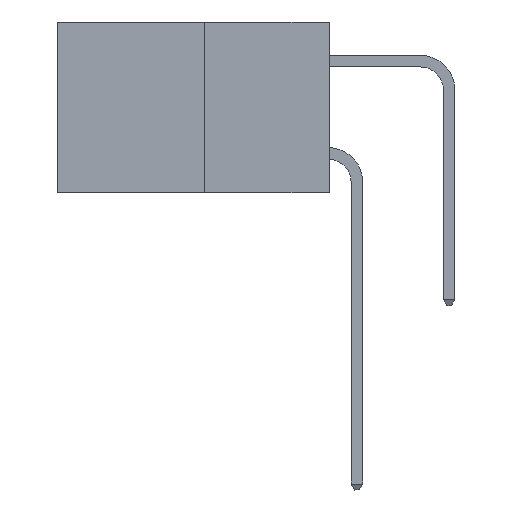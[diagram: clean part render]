
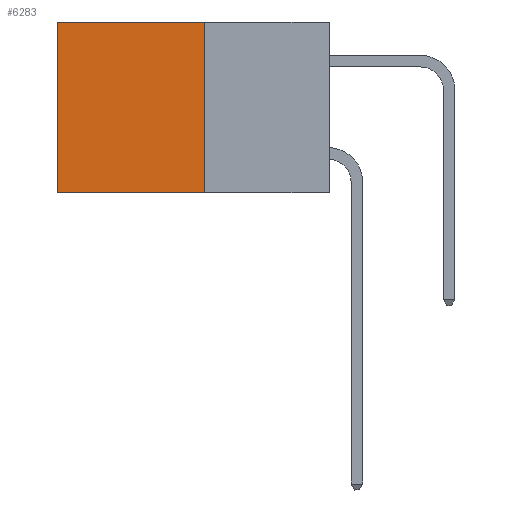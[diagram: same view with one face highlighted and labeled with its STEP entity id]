
A CAD part, left-side view. The second image highlights one B-rep face of the part: STEP entity #6283.
In plain terms, the highlighted planar face has unit normal (-1, 0, 0).
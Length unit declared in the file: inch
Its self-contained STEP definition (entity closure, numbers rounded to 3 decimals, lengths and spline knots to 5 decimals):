
#1158 = DIRECTION ( 'NONE',  ( 0., 0., -1. ) ) ;
#1162 = VERTEX_POINT ( 'NONE', #4892 ) ;
#2127 = VECTOR ( 'NONE', #2379, 39.37008 ) ;
#2379 = DIRECTION ( 'NONE',  ( 0., 0., -1. ) ) ;
#3641 = CARTESIAN_POINT ( 'NONE',  ( 0.277, 0.27, 0. ) ) ;
#4084 = CARTESIAN_POINT ( 'NONE',  ( 0.277, 0.27, 0. ) ) ;
#4225 = CARTESIAN_POINT ( 'NONE',  ( 0.277, 0.59, -0.37 ) ) ;
#4892 = CARTESIAN_POINT ( 'NONE',  ( 0.277, 0.59, 0. ) ) ;
#6283 = ADVANCED_FACE ( 'NONE', ( #9417 ), #22068, .F. ) ;
#6819 = LINE ( 'NONE', #11114, #2127 ) ;
#7286 = ORIENTED_EDGE ( 'NONE', *, *, #8334, .T. ) ;
#7299 = LINE ( 'NONE', #22049, #10817 ) ;
#7379 = ORIENTED_EDGE ( 'NONE', *, *, #16635, .F. ) ;
#7497 = CARTESIAN_POINT ( 'NONE',  ( 0.277, 0.27, -0.37 ) ) ;
#7583 = LINE ( 'NONE', #7497, #16349 ) ;
#7640 = ORIENTED_EDGE ( 'NONE', *, *, #21162, .T. ) ;
#8214 = EDGE_LOOP ( 'NONE', ( #7640, #9805, #7379, #7286 ) ) ;
#8334 = EDGE_CURVE ( 'NONE', #17222, #1162, #14246, .T. ) ;
#9417 = FACE_OUTER_BOUND ( 'NONE', #8214, .T. ) ;
#9805 = ORIENTED_EDGE ( 'NONE', *, *, #16900, .F. ) ;
#9912 = CARTESIAN_POINT ( 'NONE',  ( 0.277, 0.27, -0.37 ) ) ;
#10817 = VECTOR ( 'NONE', #22115, 39.37008 ) ;
#11114 = CARTESIAN_POINT ( 'NONE',  ( 0.277, 0.59, -0.37 ) ) ;
#11692 = DIRECTION ( 'NONE',  ( 1., 0., 0. ) ) ;
#14246 = LINE ( 'NONE', #4084, #17820 ) ;
#15899 = VERTEX_POINT ( 'NONE', #4225 ) ;
#16349 = VECTOR ( 'NONE', #21455, 39.37008 ) ;
#16635 = EDGE_CURVE ( 'NONE', #17222, #22518, #7583, .T. ) ;
#16900 = EDGE_CURVE ( 'NONE', #22518, #15899, #7299, .T. ) ;
#17222 = VERTEX_POINT ( 'NONE', #3641 ) ;
#17820 = VECTOR ( 'NONE', #19813, 39.37008 ) ;
#18425 = CARTESIAN_POINT ( 'NONE',  ( 0.277, 0.27, -0.37 ) ) ;
#18682 = AXIS2_PLACEMENT_3D ( 'NONE', #9912, #11692, #1158 ) ;
#19813 = DIRECTION ( 'NONE',  ( 0., 1., 0. ) ) ;
#21162 = EDGE_CURVE ( 'NONE', #1162, #15899, #6819, .T. ) ;
#21455 = DIRECTION ( 'NONE',  ( 0., 0., -1. ) ) ;
#22049 = CARTESIAN_POINT ( 'NONE',  ( 0.277, 0.27, -0.37 ) ) ;
#22068 = PLANE ( 'NONE',  #18682 ) ;
#22115 = DIRECTION ( 'NONE',  ( 0., 1., 0. ) ) ;
#22518 = VERTEX_POINT ( 'NONE', #18425 ) ;
